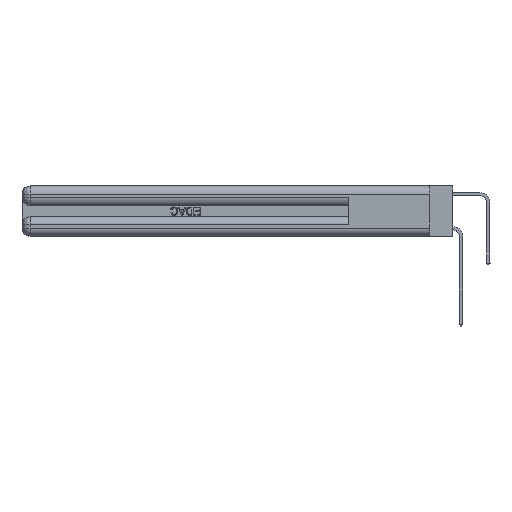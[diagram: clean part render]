
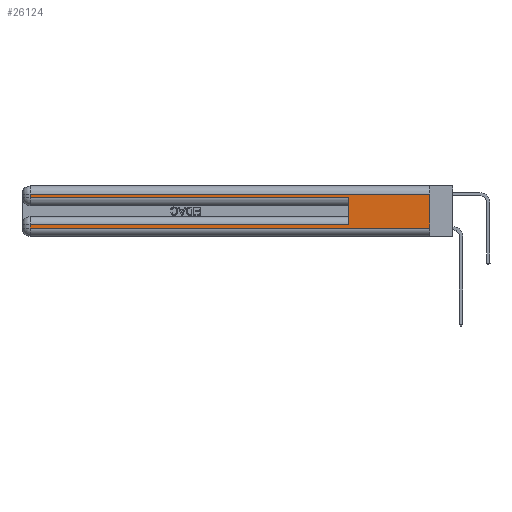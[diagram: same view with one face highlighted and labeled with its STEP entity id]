
A CAD part, left-side view. The second image highlights one B-rep face of the part: STEP entity #26124.
In plain terms, the highlighted planar face has unit normal (-1, 0, 0).
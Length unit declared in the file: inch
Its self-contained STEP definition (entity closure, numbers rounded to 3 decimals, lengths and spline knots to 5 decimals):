
#248 = VERTEX_POINT ( 'NONE', #31521 ) ;
#780 = DIRECTION ( 'NONE',  ( 0., 0., -1. ) ) ;
#1308 = DIRECTION ( 'NONE',  ( 1., 0., 0. ) ) ;
#1986 = DIRECTION ( 'NONE',  ( 0., 1., 0. ) ) ;
#2087 = EDGE_CURVE ( 'NONE', #17303, #14055, #31867, .T. ) ;
#3908 = CARTESIAN_POINT ( 'NONE',  ( 0., 2.94, 0.37 ) ) ;
#3948 = CARTESIAN_POINT ( 'NONE',  ( 0., 0., 0.37 ) ) ;
#5357 = VERTEX_POINT ( 'NONE', #16088 ) ;
#6427 = ORIENTED_EDGE ( 'NONE', *, *, #31931, .T. ) ;
#8595 = DIRECTION ( 'NONE',  ( 0., 1., 0. ) ) ;
#9071 = CARTESIAN_POINT ( 'NONE',  ( 0., 0., 0.37 ) ) ;
#9112 = VECTOR ( 'NONE', #27798, 39.37008 ) ;
#9170 = EDGE_LOOP ( 'NONE', ( #19855, #6427, #26980, #11910, #17845, #13153, #26245, #16850 ) ) ;
#9416 = CARTESIAN_POINT ( 'NONE',  ( 0., 0., 0.285 ) ) ;
#11057 = VERTEX_POINT ( 'NONE', #11866 ) ;
#11314 = VERTEX_POINT ( 'NONE', #23018 ) ;
#11866 = CARTESIAN_POINT ( 'NONE',  ( 0., 0.6, 0.085 ) ) ;
#11910 = ORIENTED_EDGE ( 'NONE', *, *, #33340, .T. ) ;
#13153 = ORIENTED_EDGE ( 'NONE', *, *, #28612, .T. ) ;
#13696 = CARTESIAN_POINT ( 'NONE',  ( 0., 0., 0.085 ) ) ;
#14055 = VERTEX_POINT ( 'NONE', #29778 ) ;
#15222 = CARTESIAN_POINT ( 'NONE',  ( 0., 2.94, 0.285 ) ) ;
#15298 = VECTOR ( 'NONE', #30290, 39.37008 ) ;
#15920 = EDGE_CURVE ( 'NONE', #5357, #14055, #24653, .T. ) ;
#16088 = CARTESIAN_POINT ( 'NONE',  ( 0., 0., 0.31 ) ) ;
#16674 = DIRECTION ( 'NONE',  ( 0., 0., -1. ) ) ;
#16850 = ORIENTED_EDGE ( 'NONE', *, *, #2087, .T. ) ;
#16989 = CARTESIAN_POINT ( 'NONE',  ( 0., 0.6, 0.145 ) ) ;
#17303 = VERTEX_POINT ( 'NONE', #19396 ) ;
#17320 = VECTOR ( 'NONE', #27571, 39.37008 ) ;
#17774 = VECTOR ( 'NONE', #8595, 39.37008 ) ;
#17845 = ORIENTED_EDGE ( 'NONE', *, *, #34918, .F. ) ;
#18243 = LINE ( 'NONE', #9416, #28356 ) ;
#18400 = CARTESIAN_POINT ( 'NONE',  ( 0., 0., 0.06 ) ) ;
#19396 = CARTESIAN_POINT ( 'NONE',  ( 0., 2.94, 0.06 ) ) ;
#19855 = ORIENTED_EDGE ( 'NONE', *, *, #15920, .F. ) ;
#19858 = LINE ( 'NONE', #30318, #27154 ) ;
#20042 = DIRECTION ( 'NONE',  ( 0., 0., -1. ) ) ;
#20739 = FACE_OUTER_BOUND ( 'NONE', #9170, .T. ) ;
#20942 = VERTEX_POINT ( 'NONE', #15222 ) ;
#21855 = LINE ( 'NONE', #13696, #17774 ) ;
#23018 = CARTESIAN_POINT ( 'NONE',  ( 0., 0.6, 0.285 ) ) ;
#23216 = LINE ( 'NONE', #33686, #28837 ) ;
#23885 = AXIS2_PLACEMENT_3D ( 'NONE', #3948, #1308, #20042 ) ;
#24653 = LINE ( 'NONE', #9071, #27025 ) ;
#26124 = ADVANCED_FACE ( 'NONE', ( #20739 ), #28182, .F. ) ;
#26245 = ORIENTED_EDGE ( 'NONE', *, *, #31805, .T. ) ;
#26980 = ORIENTED_EDGE ( 'NONE', *, *, #34905, .T. ) ;
#27025 = VECTOR ( 'NONE', #780, 39.37008 ) ;
#27154 = VECTOR ( 'NONE', #16674, 39.37008 ) ;
#27571 = DIRECTION ( 'NONE',  ( 0., -1., 0. ) ) ;
#27798 = DIRECTION ( 'NONE',  ( 0., 0., 1. ) ) ;
#28182 = PLANE ( 'NONE',  #23885 ) ;
#28356 = VECTOR ( 'NONE', #33875, 39.37008 ) ;
#28612 = EDGE_CURVE ( 'NONE', #11057, #248, #21855, .T. ) ;
#28837 = VECTOR ( 'NONE', #1986, 39.37008 ) ;
#28968 = VERTEX_POINT ( 'NONE', #30132 ) ;
#29778 = CARTESIAN_POINT ( 'NONE',  ( 0., 0., 0.06 ) ) ;
#30132 = CARTESIAN_POINT ( 'NONE',  ( 0., 2.94, 0.31 ) ) ;
#30290 = DIRECTION ( 'NONE',  ( 0., 0., -1. ) ) ;
#30318 = CARTESIAN_POINT ( 'NONE',  ( 0., 2.94, 0.37 ) ) ;
#31521 = CARTESIAN_POINT ( 'NONE',  ( 0., 2.94, 0.085 ) ) ;
#31805 = EDGE_CURVE ( 'NONE', #248, #17303, #19858, .T. ) ;
#31867 = LINE ( 'NONE', #18400, #17320 ) ;
#31931 = EDGE_CURVE ( 'NONE', #5357, #28968, #23216, .T. ) ;
#32951 = LINE ( 'NONE', #3908, #15298 ) ;
#33340 = EDGE_CURVE ( 'NONE', #20942, #11314, #18243, .T. ) ;
#33476 = LINE ( 'NONE', #16989, #9112 ) ;
#33686 = CARTESIAN_POINT ( 'NONE',  ( 0., 0., 0.31 ) ) ;
#33875 = DIRECTION ( 'NONE',  ( 0., -1., 0. ) ) ;
#34905 = EDGE_CURVE ( 'NONE', #28968, #20942, #32951, .T. ) ;
#34918 = EDGE_CURVE ( 'NONE', #11057, #11314, #33476, .T. ) ;
